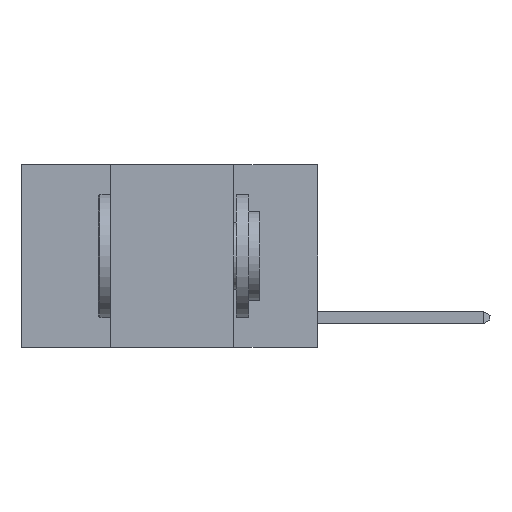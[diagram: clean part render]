
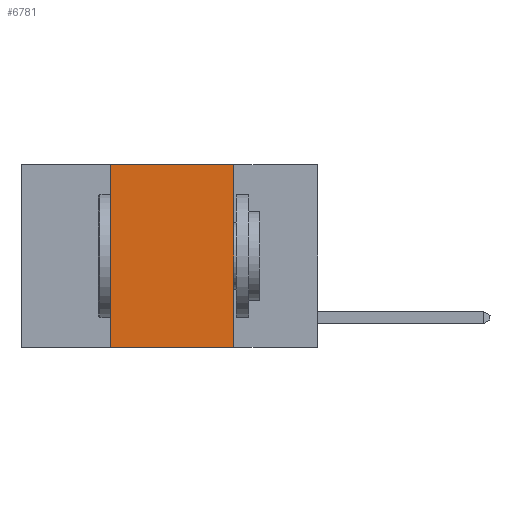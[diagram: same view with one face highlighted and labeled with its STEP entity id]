
A CAD part, left-side view. The second image highlights one B-rep face of the part: STEP entity #6781.
In plain terms, the highlighted planar face has unit normal (-1, 0, 0).
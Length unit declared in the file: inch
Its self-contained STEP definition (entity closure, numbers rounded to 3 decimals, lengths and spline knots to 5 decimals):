
#603 = VERTEX_POINT ( 'NONE', #8288 ) ;
#665 = CARTESIAN_POINT ( 'NONE',  ( 0., 0.42, 0. ) ) ;
#696 = EDGE_CURVE ( 'NONE', #20408, #4447, #5534, .T. ) ;
#986 = LINE ( 'NONE', #3977, #16141 ) ;
#1675 = VECTOR ( 'NONE', #6984, 39.37008 ) ;
#2248 = CARTESIAN_POINT ( 'NONE',  ( 0., 0.6, 0. ) ) ;
#2962 = CARTESIAN_POINT ( 'NONE',  ( 0., 0.17, -0.37 ) ) ;
#3059 = ORIENTED_EDGE ( 'NONE', *, *, #21832, .F. ) ;
#3205 = CARTESIAN_POINT ( 'NONE',  ( 0., 0.6, 0. ) ) ;
#3316 = DIRECTION ( 'NONE',  ( 1., 0., 0. ) ) ;
#3779 = ORIENTED_EDGE ( 'NONE', *, *, #18550, .F. ) ;
#3902 = LINE ( 'NONE', #2248, #16863 ) ;
#3964 = CARTESIAN_POINT ( 'NONE',  ( 0., 0.42, 0. ) ) ;
#3977 = CARTESIAN_POINT ( 'NONE',  ( 0., 0.17, 0. ) ) ;
#4447 = VERTEX_POINT ( 'NONE', #665 ) ;
#5534 = LINE ( 'NONE', #3964, #6457 ) ;
#5881 = DIRECTION ( 'NONE',  ( 0., 0., -1. ) ) ;
#6457 = VECTOR ( 'NONE', #6973, 39.37008 ) ;
#6781 = ADVANCED_FACE ( 'NONE', ( #7079 ), #17089, .F. ) ;
#6973 = DIRECTION ( 'NONE',  ( 0., 0., 1. ) ) ;
#6984 = DIRECTION ( 'NONE',  ( 0., -1., 0. ) ) ;
#7079 = FACE_OUTER_BOUND ( 'NONE', #9664, .T. ) ;
#7423 = CARTESIAN_POINT ( 'NONE',  ( 0., 0.42, -0.37 ) ) ;
#8146 = EDGE_CURVE ( 'NONE', #20408, #8480, #16988, .T. ) ;
#8288 = CARTESIAN_POINT ( 'NONE',  ( 0., 0.17, 0. ) ) ;
#8480 = VERTEX_POINT ( 'NONE', #2962 ) ;
#8745 = CARTESIAN_POINT ( 'NONE',  ( 0., 0.6, -0.37 ) ) ;
#8877 = DIRECTION ( 'NONE',  ( 0., -1., 0. ) ) ;
#9664 = EDGE_LOOP ( 'NONE', ( #3059, #3779, #11324, #19221 ) ) ;
#11324 = ORIENTED_EDGE ( 'NONE', *, *, #696, .F. ) ;
#11540 = AXIS2_PLACEMENT_3D ( 'NONE', #3205, #3316, #12113 ) ;
#12113 = DIRECTION ( 'NONE',  ( 0., 0., -1. ) ) ;
#16141 = VECTOR ( 'NONE', #5881, 39.37008 ) ;
#16863 = VECTOR ( 'NONE', #8877, 39.37008 ) ;
#16988 = LINE ( 'NONE', #8745, #1675 ) ;
#17089 = PLANE ( 'NONE',  #11540 ) ;
#18550 = EDGE_CURVE ( 'NONE', #4447, #603, #3902, .T. ) ;
#19221 = ORIENTED_EDGE ( 'NONE', *, *, #8146, .T. ) ;
#20408 = VERTEX_POINT ( 'NONE', #7423 ) ;
#21832 = EDGE_CURVE ( 'NONE', #603, #8480, #986, .T. ) ;
